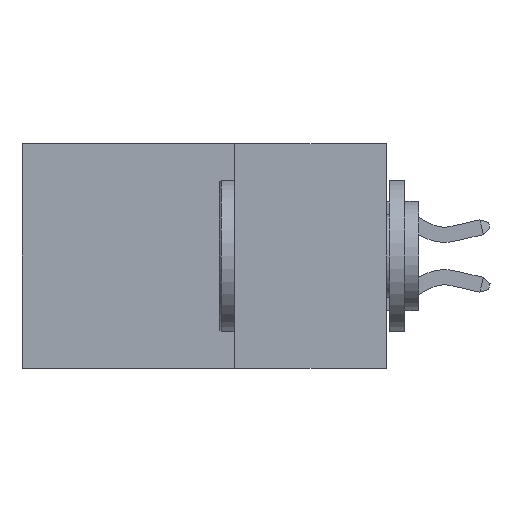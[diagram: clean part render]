
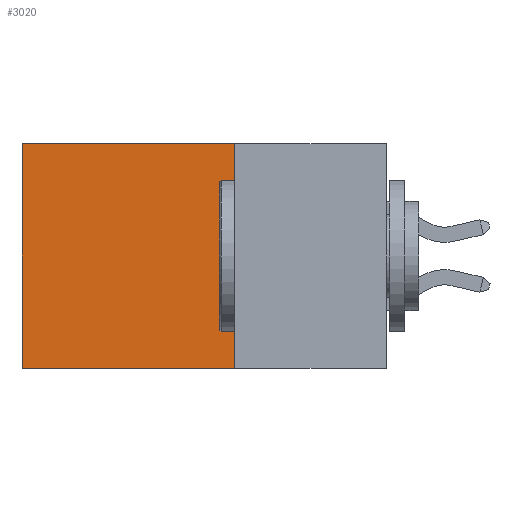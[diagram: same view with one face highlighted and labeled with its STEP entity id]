
A CAD part, left-side view. The second image highlights one B-rep face of the part: STEP entity #3020.
In plain terms, the highlighted planar face has unit normal (-1, 0, 0).
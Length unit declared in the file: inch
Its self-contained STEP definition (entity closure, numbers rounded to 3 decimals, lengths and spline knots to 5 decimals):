
#74 = ORIENTED_EDGE ( 'NONE', *, *, #15569, .T. ) ;
#97 = CARTESIAN_POINT ( 'NONE',  ( 0.298, 0.25, -0.37 ) ) ;
#1217 = PLANE ( 'NONE',  #15972 ) ;
#1559 = ORIENTED_EDGE ( 'NONE', *, *, #19271, .F. ) ;
#2800 = DIRECTION ( 'NONE',  ( 0., 0., -1. ) ) ;
#3020 = ADVANCED_FACE ( 'NONE', ( #19936 ), #1217, .F. ) ;
#3032 = DIRECTION ( 'NONE',  ( 0., 0., -1. ) ) ;
#6789 = VECTOR ( 'NONE', #2800, 39.37008 ) ;
#7330 = EDGE_CURVE ( 'NONE', #11455, #16258, #13607, .T. ) ;
#7659 = LINE ( 'NONE', #26298, #11202 ) ;
#8034 = VERTEX_POINT ( 'NONE', #26385 ) ;
#8081 = LINE ( 'NONE', #11180, #6789 ) ;
#9455 = ORIENTED_EDGE ( 'NONE', *, *, #18052, .F. ) ;
#9949 = DIRECTION ( 'NONE',  ( 0., 0., -1. ) ) ;
#11180 = CARTESIAN_POINT ( 'NONE',  ( 0.298, 0.25, 0. ) ) ;
#11202 = VECTOR ( 'NONE', #13535, 39.37008 ) ;
#11455 = VERTEX_POINT ( 'NONE', #19354 ) ;
#11979 = VECTOR ( 'NONE', #9949, 39.37008 ) ;
#13535 = DIRECTION ( 'NONE',  ( 0., 1., 0. ) ) ;
#13607 = LINE ( 'NONE', #16006, #11979 ) ;
#13882 = VECTOR ( 'NONE', #14021, 39.37008 ) ;
#14021 = DIRECTION ( 'NONE',  ( 0., 1., 0. ) ) ;
#15077 = EDGE_LOOP ( 'NONE', ( #25754, #1559, #9455, #74 ) ) ;
#15569 = EDGE_CURVE ( 'NONE', #8034, #11455, #19364, .T. ) ;
#15972 = AXIS2_PLACEMENT_3D ( 'NONE', #17515, #25910, #3032 ) ;
#16006 = CARTESIAN_POINT ( 'NONE',  ( 0.298, 0.6, 0. ) ) ;
#16258 = VERTEX_POINT ( 'NONE', #21329 ) ;
#17515 = CARTESIAN_POINT ( 'NONE',  ( 0.298, 0.25, 0. ) ) ;
#18052 = EDGE_CURVE ( 'NONE', #8034, #21536, #8081, .T. ) ;
#18177 = CARTESIAN_POINT ( 'NONE',  ( 0.298, 0.25, 0. ) ) ;
#19271 = EDGE_CURVE ( 'NONE', #21536, #16258, #7659, .T. ) ;
#19354 = CARTESIAN_POINT ( 'NONE',  ( 0.298, 0.6, 0. ) ) ;
#19364 = LINE ( 'NONE', #18177, #13882 ) ;
#19936 = FACE_OUTER_BOUND ( 'NONE', #15077, .T. ) ;
#21329 = CARTESIAN_POINT ( 'NONE',  ( 0.298, 0.6, -0.37 ) ) ;
#21536 = VERTEX_POINT ( 'NONE', #97 ) ;
#25754 = ORIENTED_EDGE ( 'NONE', *, *, #7330, .T. ) ;
#25910 = DIRECTION ( 'NONE',  ( 1., 0., 0. ) ) ;
#26298 = CARTESIAN_POINT ( 'NONE',  ( 0.298, 0.25, -0.37 ) ) ;
#26385 = CARTESIAN_POINT ( 'NONE',  ( 0.298, 0.25, 0. ) ) ;
